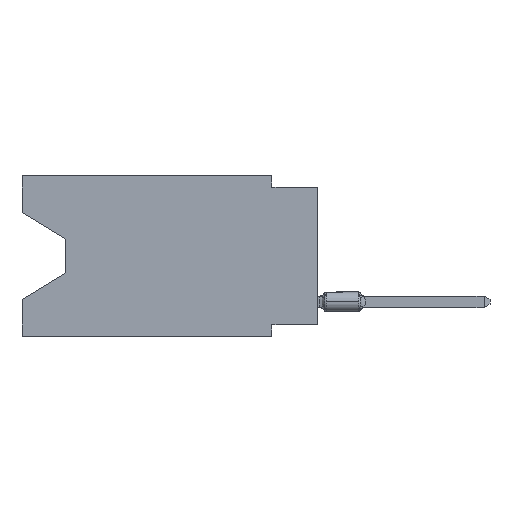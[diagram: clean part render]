
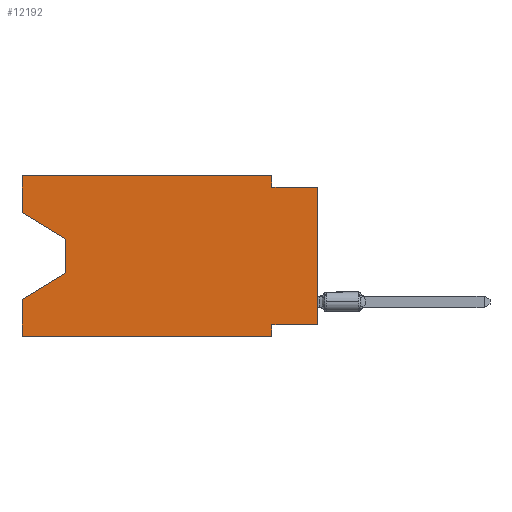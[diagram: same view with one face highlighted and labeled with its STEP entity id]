
A CAD part, left-side view. The second image highlights one B-rep face of the part: STEP entity #12192.
In plain terms, the highlighted planar face has unit normal (-1, 0, 0).
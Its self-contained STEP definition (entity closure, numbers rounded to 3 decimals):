
#12 = EDGE_CURVE ( 'NONE', #7865, #8941, #2552, .T. ) ;
#83 = DIRECTION ( 'NONE',  ( 0., 0., -1. ) ) ;
#504 = VECTOR ( 'NONE', #5763, 1000. ) ;
#792 = EDGE_CURVE ( 'NONE', #7865, #15329, #971, .T. ) ;
#877 = VECTOR ( 'NONE', #83, 1000. ) ;
#889 = PLANE ( 'NONE',  #13996 ) ;
#971 = LINE ( 'NONE', #17600, #2901 ) ;
#1103 = LINE ( 'NONE', #19228, #14267 ) ;
#1123 = ORIENTED_EDGE ( 'NONE', *, *, #16195, .F. ) ;
#1388 = EDGE_CURVE ( 'NONE', #16147, #3523, #19498, .T. ) ;
#1754 = DIRECTION ( 'NONE',  ( 0., 0., -1. ) ) ;
#1821 = ORIENTED_EDGE ( 'NONE', *, *, #16404, .F. ) ;
#2116 = ORIENTED_EDGE ( 'NONE', *, *, #12, .T. ) ;
#2481 = DIRECTION ( 'NONE',  ( 0., 0., 1. ) ) ;
#2552 = LINE ( 'NONE', #4361, #504 ) ;
#2891 = LINE ( 'NONE', #15884, #13277 ) ;
#2901 = VECTOR ( 'NONE', #2481, 1000. ) ;
#3076 = CARTESIAN_POINT ( 'NONE',  ( 0., 13.97, -3.505 ) ) ;
#3078 = LINE ( 'NONE', #21002, #4409 ) ;
#3346 = VERTEX_POINT ( 'NONE', #3076 ) ;
#3349 = CARTESIAN_POINT ( 'NONE',  ( 0., 13.97, -3.505 ) ) ;
#3523 = VERTEX_POINT ( 'NONE', #16492 ) ;
#3799 = CARTESIAN_POINT ( 'NONE',  ( 0., 16.383, 0. ) ) ;
#4361 = CARTESIAN_POINT ( 'NONE',  ( 0., 16.383, -8.89 ) ) ;
#4409 = VECTOR ( 'NONE', #16061, 1000. ) ;
#4634 = LINE ( 'NONE', #11173, #12936 ) ;
#5017 = VERTEX_POINT ( 'NONE', #14849 ) ;
#5258 = EDGE_CURVE ( 'NONE', #12411, #5280, #1103, .T. ) ;
#5280 = VERTEX_POINT ( 'NONE', #6337 ) ;
#5763 = DIRECTION ( 'NONE',  ( 0., -1., 0. ) ) ;
#6018 = CARTESIAN_POINT ( 'NONE',  ( 0., 0., -8.255 ) ) ;
#6020 = ORIENTED_EDGE ( 'NONE', *, *, #6804, .F. ) ;
#6337 = CARTESIAN_POINT ( 'NONE',  ( 0., 0., -0.635 ) ) ;
#6662 = CARTESIAN_POINT ( 'NONE',  ( 0., 2.54, -8.89 ) ) ;
#6804 = EDGE_CURVE ( 'NONE', #13239, #16147, #8243, .T. ) ;
#7008 = FACE_OUTER_BOUND ( 'NONE', #12524, .T. ) ;
#7778 = VECTOR ( 'NONE', #9132, 1000. ) ;
#7865 = VERTEX_POINT ( 'NONE', #12683 ) ;
#7909 = CARTESIAN_POINT ( 'NONE',  ( 0., 16.383, 0. ) ) ;
#7970 = EDGE_CURVE ( 'NONE', #3346, #19345, #11613, .T. ) ;
#8040 = EDGE_CURVE ( 'NONE', #18533, #8941, #16456, .T. ) ;
#8158 = VECTOR ( 'NONE', #19736, 1000. ) ;
#8219 = CARTESIAN_POINT ( 'NONE',  ( 0., 2.54, 0. ) ) ;
#8243 = LINE ( 'NONE', #13180, #8158 ) ;
#8941 = VERTEX_POINT ( 'NONE', #18507 ) ;
#9111 = DIRECTION ( 'NONE',  ( 0., -1., 0. ) ) ;
#9132 = DIRECTION ( 'NONE',  ( 0., 1., 0. ) ) ;
#9378 = CARTESIAN_POINT ( 'NONE',  ( 0., 2.54, -8.255 ) ) ;
#9404 = CARTESIAN_POINT ( 'NONE',  ( 0., 13.97, -5.385 ) ) ;
#9522 = ORIENTED_EDGE ( 'NONE', *, *, #11455, .F. ) ;
#9552 = ORIENTED_EDGE ( 'NONE', *, *, #7970, .T. ) ;
#11173 = CARTESIAN_POINT ( 'NONE',  ( 0., 13.97, -5.385 ) ) ;
#11399 = LINE ( 'NONE', #13430, #11561 ) ;
#11455 = EDGE_CURVE ( 'NONE', #3523, #5280, #2891, .T. ) ;
#11561 = VECTOR ( 'NONE', #16651, 1000. ) ;
#11613 = LINE ( 'NONE', #3349, #20995 ) ;
#12192 = ADVANCED_FACE ( 'NONE', ( #7008 ), #889, .F. ) ;
#12411 = VERTEX_POINT ( 'NONE', #15046 ) ;
#12433 = ORIENTED_EDGE ( 'NONE', *, *, #14189, .T. ) ;
#12524 = EDGE_LOOP ( 'NONE', ( #12433, #9552, #18152, #14146, #2116, #18616, #1123, #18439, #9522, #13414, #6020, #1821 ) ) ;
#12530 = CARTESIAN_POINT ( 'NONE',  ( 0., 16.383, -6.852 ) ) ;
#12683 = CARTESIAN_POINT ( 'NONE',  ( 0., 16.383, -8.89 ) ) ;
#12936 = VECTOR ( 'NONE', #19552, 1000. ) ;
#13180 = CARTESIAN_POINT ( 'NONE',  ( 0., 16.383, 0. ) ) ;
#13239 = VERTEX_POINT ( 'NONE', #7909 ) ;
#13277 = VECTOR ( 'NONE', #9111, 1000. ) ;
#13414 = ORIENTED_EDGE ( 'NONE', *, *, #1388, .F. ) ;
#13430 = CARTESIAN_POINT ( 'NONE',  ( 0., 16.383, 0. ) ) ;
#13861 = CARTESIAN_POINT ( 'NONE',  ( 0., 2.54, 0. ) ) ;
#13975 = DIRECTION ( 'NONE',  ( 1., 0., 0. ) ) ;
#13996 = AXIS2_PLACEMENT_3D ( 'NONE', #3799, #13975, #15386 ) ;
#14146 = ORIENTED_EDGE ( 'NONE', *, *, #792, .F. ) ;
#14189 = EDGE_CURVE ( 'NONE', #5017, #3346, #3078, .T. ) ;
#14267 = VECTOR ( 'NONE', #15901, 1000. ) ;
#14516 = DIRECTION ( 'NONE',  ( 0., 0., -1. ) ) ;
#14849 = CARTESIAN_POINT ( 'NONE',  ( 0., 16.383, -2.038 ) ) ;
#15046 = CARTESIAN_POINT ( 'NONE',  ( 0., 0., -8.255 ) ) ;
#15329 = VERTEX_POINT ( 'NONE', #12530 ) ;
#15386 = DIRECTION ( 'NONE',  ( 0., 0., -1. ) ) ;
#15884 = CARTESIAN_POINT ( 'NONE',  ( 0., 0., -0.635 ) ) ;
#15901 = DIRECTION ( 'NONE',  ( 0., 0., 1. ) ) ;
#16061 = DIRECTION ( 'NONE',  ( 0., -0.855, -0.519 ) ) ;
#16147 = VERTEX_POINT ( 'NONE', #13861 ) ;
#16195 = EDGE_CURVE ( 'NONE', #12411, #18533, #19122, .T. ) ;
#16201 = VECTOR ( 'NONE', #1754, 1000. ) ;
#16302 = EDGE_CURVE ( 'NONE', #19345, #15329, #4634, .T. ) ;
#16404 = EDGE_CURVE ( 'NONE', #5017, #13239, #11399, .T. ) ;
#16456 = LINE ( 'NONE', #6662, #16201 ) ;
#16492 = CARTESIAN_POINT ( 'NONE',  ( 0., 2.54, -0.635 ) ) ;
#16651 = DIRECTION ( 'NONE',  ( 0., 0., 1. ) ) ;
#17600 = CARTESIAN_POINT ( 'NONE',  ( 0., 16.383, 0. ) ) ;
#18152 = ORIENTED_EDGE ( 'NONE', *, *, #16302, .T. ) ;
#18439 = ORIENTED_EDGE ( 'NONE', *, *, #5258, .T. ) ;
#18507 = CARTESIAN_POINT ( 'NONE',  ( 0., 2.54, -8.89 ) ) ;
#18533 = VERTEX_POINT ( 'NONE', #9378 ) ;
#18616 = ORIENTED_EDGE ( 'NONE', *, *, #8040, .F. ) ;
#19122 = LINE ( 'NONE', #6018, #7778 ) ;
#19228 = CARTESIAN_POINT ( 'NONE',  ( 0., 0., 0. ) ) ;
#19345 = VERTEX_POINT ( 'NONE', #9404 ) ;
#19498 = LINE ( 'NONE', #8219, #877 ) ;
#19552 = DIRECTION ( 'NONE',  ( 0., 0.855, -0.519 ) ) ;
#19736 = DIRECTION ( 'NONE',  ( 0., -1., 0. ) ) ;
#20995 = VECTOR ( 'NONE', #14516, 1000. ) ;
#21002 = CARTESIAN_POINT ( 'NONE',  ( 0., 16.383, -2.038 ) ) ;
